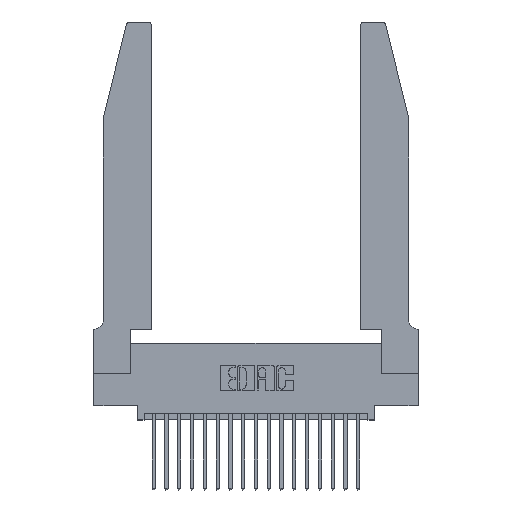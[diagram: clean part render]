
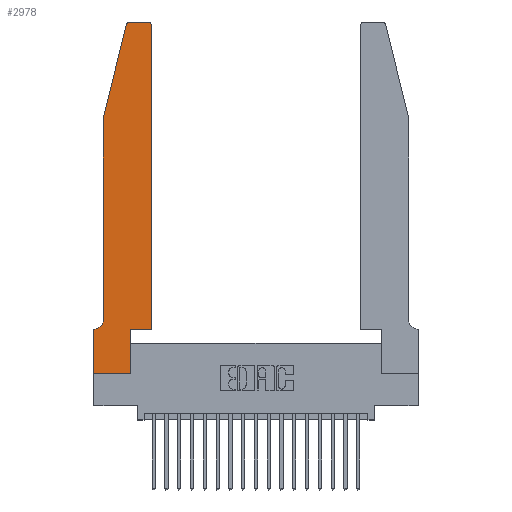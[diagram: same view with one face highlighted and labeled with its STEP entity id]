
A CAD part, top view. The second image highlights one B-rep face of the part: STEP entity #2978.
In plain terms, the highlighted planar face has unit normal (0, 0, 1).
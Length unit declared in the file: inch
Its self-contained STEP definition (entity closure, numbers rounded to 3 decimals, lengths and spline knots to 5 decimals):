
#91 = LINE ( 'NONE', #20828, #15750 ) ;
#445 = DIRECTION ( 'NONE',  ( 0., 0., 1. ) ) ;
#815 = VERTEX_POINT ( 'NONE', #16757 ) ;
#834 = VERTEX_POINT ( 'NONE', #13384 ) ;
#839 = DIRECTION ( 'NONE',  ( 0., 1., 0. ) ) ;
#1062 = EDGE_CURVE ( 'NONE', #16441, #815, #19193, .T. ) ;
#1763 = VERTEX_POINT ( 'NONE', #15951 ) ;
#1841 = VERTEX_POINT ( 'NONE', #11842 ) ;
#1993 = VERTEX_POINT ( 'NONE', #3700 ) ;
#2141 = EDGE_CURVE ( 'NONE', #1993, #8886, #13127, .T. ) ;
#2334 = CARTESIAN_POINT ( 'NONE',  ( 0., 0., 0.37 ) ) ;
#2964 = ORIENTED_EDGE ( 'NONE', *, *, #19640, .T. ) ;
#2978 = ADVANCED_FACE ( 'NONE', ( #15176 ), #3583, .T. ) ;
#3381 = CARTESIAN_POINT ( 'NONE',  ( 0., 0.35, 0.37 ) ) ;
#3428 = LINE ( 'NONE', #18513, #10146 ) ;
#3583 = PLANE ( 'NONE',  #17399 ) ;
#3589 = CIRCLE ( 'NONE', #13459, 0.03 ) ;
#3700 = CARTESIAN_POINT ( 'NONE',  ( 0., 0., 0.37 ) ) ;
#4039 = CARTESIAN_POINT ( 'NONE',  ( 0.2865, 0., 0.37 ) ) ;
#4218 = EDGE_CURVE ( 'NONE', #815, #10964, #91, .T. ) ;
#4948 = LINE ( 'NONE', #10450, #7791 ) ;
#5153 = DIRECTION ( 'NONE',  ( 0., 0., -1. ) ) ;
#5306 = VECTOR ( 'NONE', #17193, 39.37008 ) ;
#5590 = CARTESIAN_POINT ( 'NONE',  ( 0., 0.35, 0.37 ) ) ;
#5674 = DIRECTION ( 'NONE',  ( 0., -1., 0. ) ) ;
#6063 = CARTESIAN_POINT ( 'NONE',  ( 0.284, 2.72, 0.37 ) ) ;
#6403 = LINE ( 'NONE', #10342, #21299 ) ;
#6718 = EDGE_LOOP ( 'NONE', ( #17314, #2964, #10143, #13419, #15348, #7982, #7720, #10884, #7213, #15237, #18697, #16952 ) ) ;
#6812 = DIRECTION ( 'NONE',  ( -1., 0., 0. ) ) ;
#7213 = ORIENTED_EDGE ( 'NONE', *, *, #17757, .T. ) ;
#7262 = LINE ( 'NONE', #19433, #8033 ) ;
#7420 = CARTESIAN_POINT ( 'NONE',  ( 0.4505, 2.72, 0.37 ) ) ;
#7592 = EDGE_CURVE ( 'NONE', #15761, #1763, #7262, .T. ) ;
#7720 = ORIENTED_EDGE ( 'NONE', *, *, #8295, .T. ) ;
#7734 = DIRECTION ( 'NONE',  ( 0., 0., 1. ) ) ;
#7791 = VECTOR ( 'NONE', #18803, 39.37008 ) ;
#7982 = ORIENTED_EDGE ( 'NONE', *, *, #17477, .T. ) ;
#8033 = VECTOR ( 'NONE', #17714, 39.37008 ) ;
#8068 = VECTOR ( 'NONE', #13357, 39.37008 ) ;
#8126 = CARTESIAN_POINT ( 'NONE',  ( 0.0755, 0.35, 0.37 ) ) ;
#8295 = EDGE_CURVE ( 'NONE', #9119, #1993, #9826, .T. ) ;
#8798 = CIRCLE ( 'NONE', #11332, 0.03 ) ;
#8863 = CARTESIAN_POINT ( 'NONE',  ( 0.4505, 0.35, 0.37 ) ) ;
#8886 = VERTEX_POINT ( 'NONE', #4039 ) ;
#9119 = VERTEX_POINT ( 'NONE', #5590 ) ;
#9280 = EDGE_CURVE ( 'NONE', #834, #18277, #6403, .T. ) ;
#9826 = LINE ( 'NONE', #16164, #16100 ) ;
#10143 = ORIENTED_EDGE ( 'NONE', *, *, #9280, .T. ) ;
#10146 = VECTOR ( 'NONE', #15350, 39.37008 ) ;
#10342 = CARTESIAN_POINT ( 'NONE',  ( 0.0755, 2., 0.37 ) ) ;
#10387 = EDGE_CURVE ( 'NONE', #1841, #17400, #10923, .T. ) ;
#10450 = CARTESIAN_POINT ( 'NONE',  ( 0.2865, 0.35, 0.37 ) ) ;
#10884 = ORIENTED_EDGE ( 'NONE', *, *, #2141, .T. ) ;
#10923 = CIRCLE ( 'NONE', #14965, 0.07 ) ;
#10964 = VERTEX_POINT ( 'NONE', #7420 ) ;
#11031 = DIRECTION ( 'NONE',  ( 1., 0., 0. ) ) ;
#11332 = AXIS2_PLACEMENT_3D ( 'NONE', #18611, #445, #13804 ) ;
#11842 = CARTESIAN_POINT ( 'NONE',  ( 0.0755, 0.42, 0.37 ) ) ;
#11912 = CARTESIAN_POINT ( 'NONE',  ( 0.2865, 0.35, 0.37 ) ) ;
#12548 = LINE ( 'NONE', #8126, #8068 ) ;
#13050 = CARTESIAN_POINT ( 'NONE',  ( 0.0055, 0.35, 0.37 ) ) ;
#13127 = LINE ( 'NONE', #2334, #21475 ) ;
#13357 = DIRECTION ( 'NONE',  ( -1., 0., 0. ) ) ;
#13384 = CARTESIAN_POINT ( 'NONE',  ( 0.25487, 2.72718, 0.37 ) ) ;
#13419 = ORIENTED_EDGE ( 'NONE', *, *, #17623, .T. ) ;
#13459 = AXIS2_PLACEMENT_3D ( 'NONE', #6063, #7734, #11031 ) ;
#13804 = DIRECTION ( 'NONE',  ( 1., 0., 0. ) ) ;
#14965 = AXIS2_PLACEMENT_3D ( 'NONE', #15144, #5153, #6812 ) ;
#15144 = CARTESIAN_POINT ( 'NONE',  ( 0.0055, 0.42, 0.37 ) ) ;
#15176 = FACE_OUTER_BOUND ( 'NONE', #6718, .T. ) ;
#15224 = DIRECTION ( 'NONE',  ( 0., 0., 1. ) ) ;
#15237 = ORIENTED_EDGE ( 'NONE', *, *, #1062, .T. ) ;
#15243 = DIRECTION ( 'NONE',  ( -0.239, -0.971, 0. ) ) ;
#15348 = ORIENTED_EDGE ( 'NONE', *, *, #10387, .T. ) ;
#15350 = DIRECTION ( 'NONE',  ( 0., -1., 0. ) ) ;
#15750 = VECTOR ( 'NONE', #839, 39.37008 ) ;
#15761 = VERTEX_POINT ( 'NONE', #17160 ) ;
#15951 = CARTESIAN_POINT ( 'NONE',  ( 0.284, 2.75, 0.37 ) ) ;
#16100 = VECTOR ( 'NONE', #5674, 39.37008 ) ;
#16164 = CARTESIAN_POINT ( 'NONE',  ( 0., 0., 0.37 ) ) ;
#16441 = VERTEX_POINT ( 'NONE', #11912 ) ;
#16757 = CARTESIAN_POINT ( 'NONE',  ( 0.4505, 0.35, 0.37 ) ) ;
#16899 = DIRECTION ( 'NONE',  ( 1., 0., 0. ) ) ;
#16952 = ORIENTED_EDGE ( 'NONE', *, *, #18746, .T. ) ;
#17160 = CARTESIAN_POINT ( 'NONE',  ( 0.4205, 2.75, 0.37 ) ) ;
#17193 = DIRECTION ( 'NONE',  ( 1., 0., 0. ) ) ;
#17314 = ORIENTED_EDGE ( 'NONE', *, *, #7592, .T. ) ;
#17399 = AXIS2_PLACEMENT_3D ( 'NONE', #3381, #15224, #16899 ) ;
#17400 = VERTEX_POINT ( 'NONE', #13050 ) ;
#17477 = EDGE_CURVE ( 'NONE', #17400, #9119, #12548, .T. ) ;
#17623 = EDGE_CURVE ( 'NONE', #18277, #1841, #3428, .T. ) ;
#17714 = DIRECTION ( 'NONE',  ( -1., 0., 0. ) ) ;
#17757 = EDGE_CURVE ( 'NONE', #8886, #16441, #4948, .T. ) ;
#18277 = VERTEX_POINT ( 'NONE', #20760 ) ;
#18513 = CARTESIAN_POINT ( 'NONE',  ( 0.0755, 2., 0.37 ) ) ;
#18611 = CARTESIAN_POINT ( 'NONE',  ( 0.4205, 2.72, 0.37 ) ) ;
#18697 = ORIENTED_EDGE ( 'NONE', *, *, #4218, .T. ) ;
#18746 = EDGE_CURVE ( 'NONE', #10964, #15761, #8798, .T. ) ;
#18803 = DIRECTION ( 'NONE',  ( 0., 1., 0. ) ) ;
#19106 = DIRECTION ( 'NONE',  ( 1., 0., 0. ) ) ;
#19193 = LINE ( 'NONE', #8863, #5306 ) ;
#19433 = CARTESIAN_POINT ( 'NONE',  ( 0.2605, 2.75, 0.37 ) ) ;
#19640 = EDGE_CURVE ( 'NONE', #1763, #834, #3589, .T. ) ;
#20760 = CARTESIAN_POINT ( 'NONE',  ( 0.0755, 2., 0.37 ) ) ;
#20828 = CARTESIAN_POINT ( 'NONE',  ( 0.4505, 0.35, 0.37 ) ) ;
#21299 = VECTOR ( 'NONE', #15243, 39.37008 ) ;
#21475 = VECTOR ( 'NONE', #19106, 39.37008 ) ;
